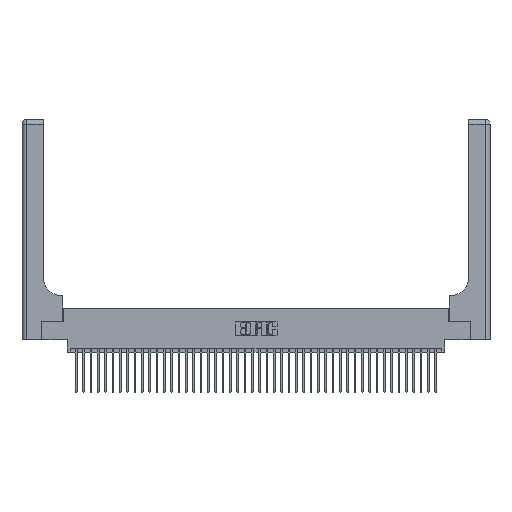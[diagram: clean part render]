
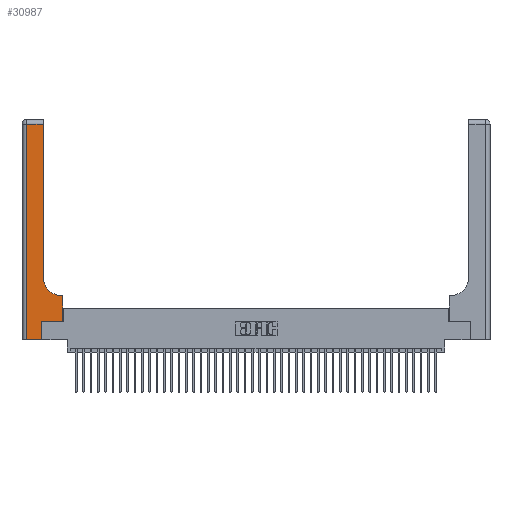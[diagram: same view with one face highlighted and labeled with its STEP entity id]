
A CAD part, top view. The second image highlights one B-rep face of the part: STEP entity #30987.
In plain terms, the highlighted planar face has unit normal (0, 0, 1).
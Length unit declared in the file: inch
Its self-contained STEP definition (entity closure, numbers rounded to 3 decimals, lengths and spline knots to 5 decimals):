
#221 = CARTESIAN_POINT ( 'NONE',  ( 0., 3., 0.37 ) ) ;
#371 = DIRECTION ( 'NONE',  ( -1., 0., 0. ) ) ;
#1116 = DIRECTION ( 'NONE',  ( 0., -1., 0. ) ) ;
#1854 = DIRECTION ( 'NONE',  ( 0., 1., 0. ) ) ;
#2064 = LINE ( 'NONE', #18017, #37838 ) ;
#2455 = EDGE_CURVE ( 'NONE', #42069, #27479, #31545, .T. ) ;
#4420 = VERTEX_POINT ( 'NONE', #19299 ) ;
#4433 = CARTESIAN_POINT ( 'NONE',  ( 0., 2.94, 0.37 ) ) ;
#5321 = ORIENTED_EDGE ( 'NONE', *, *, #31309, .T. ) ;
#5809 = CARTESIAN_POINT ( 'NONE',  ( 0., 0., 0.37 ) ) ;
#5825 = ORIENTED_EDGE ( 'NONE', *, *, #16242, .T. ) ;
#6125 = DIRECTION ( 'NONE',  ( 0., 1., 0. ) ) ;
#6269 = CARTESIAN_POINT ( 'NONE',  ( 0.2915, 3., 0.37 ) ) ;
#6319 = EDGE_CURVE ( 'NONE', #6648, #42069, #35471, .T. ) ;
#6648 = VERTEX_POINT ( 'NONE', #42336 ) ;
#10707 = DIRECTION ( 'NONE',  ( 0., 0., -1. ) ) ;
#10987 = CARTESIAN_POINT ( 'NONE',  ( 0.5585, 0.25, 0.37 ) ) ;
#11208 = EDGE_CURVE ( 'NONE', #11584, #33216, #24752, .T. ) ;
#11584 = VERTEX_POINT ( 'NONE', #34609 ) ;
#13907 = PLANE ( 'NONE',  #19221 ) ;
#14694 = DIRECTION ( 'NONE',  ( -1., 0., 0. ) ) ;
#16242 = EDGE_CURVE ( 'NONE', #33241, #36885, #2064, .T. ) ;
#17493 = CARTESIAN_POINT ( 'NONE',  ( 0.06, 0., 0.37 ) ) ;
#17583 = CARTESIAN_POINT ( 'NONE',  ( 0.5585, 0.25, 0.37 ) ) ;
#17721 = CARTESIAN_POINT ( 'NONE',  ( 0.06, 2.94, 0.37 ) ) ;
#18017 = CARTESIAN_POINT ( 'NONE',  ( 0.06, 3., 0.37 ) ) ;
#18750 = CARTESIAN_POINT ( 'NONE',  ( 0.269, 0., 0.37 ) ) ;
#19221 = AXIS2_PLACEMENT_3D ( 'NONE', #221, #20677, #371 ) ;
#19299 = CARTESIAN_POINT ( 'NONE',  ( 0.5585, 0.6, 0.37 ) ) ;
#20677 = DIRECTION ( 'NONE',  ( 0., 0., -1. ) ) ;
#21329 = FACE_OUTER_BOUND ( 'NONE', #40114, .T. ) ;
#22006 = CARTESIAN_POINT ( 'NONE',  ( 0.269, 0., 0.37 ) ) ;
#22269 = ORIENTED_EDGE ( 'NONE', *, *, #35399, .T. ) ;
#22565 = CARTESIAN_POINT ( 'NONE',  ( 0.269, 0.25, 0.37 ) ) ;
#22639 = ORIENTED_EDGE ( 'NONE', *, *, #6319, .T. ) ;
#22905 = ORIENTED_EDGE ( 'NONE', *, *, #2455, .T. ) ;
#23385 = EDGE_CURVE ( 'NONE', #4420, #6648, #40093, .T. ) ;
#23588 = AXIS2_PLACEMENT_3D ( 'NONE', #30867, #10707, #34202 ) ;
#24752 = LINE ( 'NONE', #22565, #41395 ) ;
#25933 = DIRECTION ( 'NONE',  ( 1., 0., 0. ) ) ;
#26055 = EDGE_CURVE ( 'NONE', #27479, #33241, #27969, .T. ) ;
#27034 = ORIENTED_EDGE ( 'NONE', *, *, #11208, .T. ) ;
#27234 = VECTOR ( 'NONE', #36113, 39.37008 ) ;
#27479 = VERTEX_POINT ( 'NONE', #33521 ) ;
#27752 = ORIENTED_EDGE ( 'NONE', *, *, #41374, .T. ) ;
#27805 = DIRECTION ( 'NONE',  ( 0., 1., 0. ) ) ;
#27969 = LINE ( 'NONE', #4433, #35781 ) ;
#29268 = ORIENTED_EDGE ( 'NONE', *, *, #23385, .T. ) ;
#29867 = VECTOR ( 'NONE', #27805, 39.37008 ) ;
#30212 = VECTOR ( 'NONE', #31285, 39.37008 ) ;
#30867 = CARTESIAN_POINT ( 'NONE',  ( 0.5415, 0.85, 0.37 ) ) ;
#30987 = ADVANCED_FACE ( 'NONE', ( #21329 ), #13907, .F. ) ;
#31285 = DIRECTION ( 'NONE',  ( -1., 0., 0. ) ) ;
#31309 = EDGE_CURVE ( 'NONE', #35792, #11584, #35417, .T. ) ;
#31545 = LINE ( 'NONE', #6269, #39376 ) ;
#33216 = VERTEX_POINT ( 'NONE', #17583 ) ;
#33241 = VERTEX_POINT ( 'NONE', #17721 ) ;
#33521 = CARTESIAN_POINT ( 'NONE',  ( 0.2915, 2.94, 0.37 ) ) ;
#34202 = DIRECTION ( 'NONE',  ( 1., 0., 0. ) ) ;
#34367 = CARTESIAN_POINT ( 'NONE',  ( 0.2915, 0.85, 0.37 ) ) ;
#34609 = CARTESIAN_POINT ( 'NONE',  ( 0.269, 0.25, 0.37 ) ) ;
#35399 = EDGE_CURVE ( 'NONE', #36885, #35792, #37115, .T. ) ;
#35417 = LINE ( 'NONE', #18750, #43182 ) ;
#35471 = CIRCLE ( 'NONE', #23588, 0.25 ) ;
#35781 = VECTOR ( 'NONE', #14694, 39.37008 ) ;
#35792 = VERTEX_POINT ( 'NONE', #22006 ) ;
#36113 = DIRECTION ( 'NONE',  ( 1., 0., 0. ) ) ;
#36885 = VERTEX_POINT ( 'NONE', #17493 ) ;
#37115 = LINE ( 'NONE', #5809, #27234 ) ;
#37241 = ORIENTED_EDGE ( 'NONE', *, *, #26055, .T. ) ;
#37829 = CARTESIAN_POINT ( 'NONE',  ( 0.2915, 0.6, 0.37 ) ) ;
#37838 = VECTOR ( 'NONE', #1116, 39.37008 ) ;
#39376 = VECTOR ( 'NONE', #6125, 39.37008 ) ;
#40093 = LINE ( 'NONE', #37829, #30212 ) ;
#40114 = EDGE_LOOP ( 'NONE', ( #22905, #37241, #5825, #22269, #5321, #27034, #27752, #29268, #22639 ) ) ;
#40795 = LINE ( 'NONE', #10987, #29867 ) ;
#41374 = EDGE_CURVE ( 'NONE', #33216, #4420, #40795, .T. ) ;
#41395 = VECTOR ( 'NONE', #25933, 39.37008 ) ;
#42069 = VERTEX_POINT ( 'NONE', #34367 ) ;
#42336 = CARTESIAN_POINT ( 'NONE',  ( 0.5415, 0.6, 0.37 ) ) ;
#43182 = VECTOR ( 'NONE', #1854, 39.37008 ) ;
